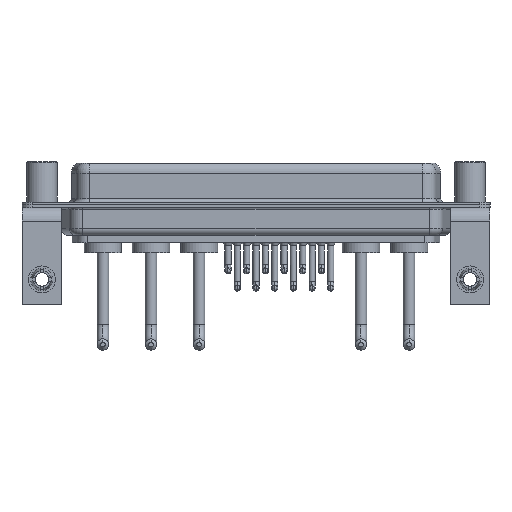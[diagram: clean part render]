
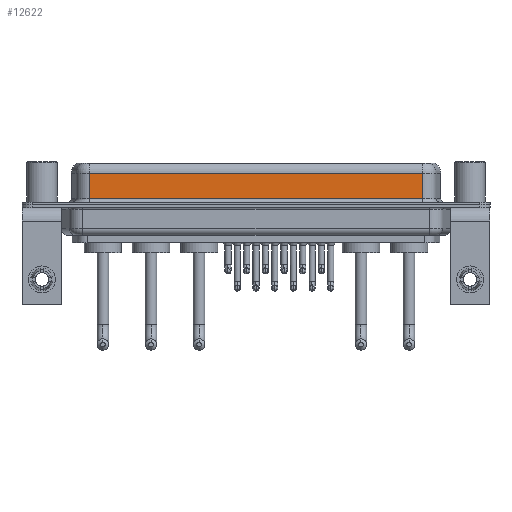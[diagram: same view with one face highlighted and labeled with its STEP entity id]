
A CAD part, front view. The second image highlights one B-rep face of the part: STEP entity #12622.
In plain terms, the highlighted planar face has unit normal (0, -1, 0).
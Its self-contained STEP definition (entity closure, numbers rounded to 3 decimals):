
#1350 = PLANE ( 'NONE',  #12972 ) ;
#1439 = ORIENTED_EDGE ( 'NONE', *, *, #18335, .T. ) ;
#1693 = CARTESIAN_POINT ( 'NONE',  ( 56.462, -3.95, 6.4 ) ) ;
#1895 = ORIENTED_EDGE ( 'NONE', *, *, #17856, .F. ) ;
#3363 = ORIENTED_EDGE ( 'NONE', *, *, #7314, .T. ) ;
#4393 = DIRECTION ( 'NONE',  ( -1., 0., 0. ) ) ;
#5036 = FACE_OUTER_BOUND ( 'NONE', #7839, .T. ) ;
#5553 = ORIENTED_EDGE ( 'NONE', *, *, #11568, .T. ) ;
#7024 = DIRECTION ( 'NONE',  ( 0., 0., 1. ) ) ;
#7314 = EDGE_CURVE ( 'NONE', #15462, #13961, #13745, .T. ) ;
#7839 = EDGE_LOOP ( 'NONE', ( #1895, #3363, #1439, #5553 ) ) ;
#8731 = VERTEX_POINT ( 'NONE', #11573 ) ;
#8867 = CARTESIAN_POINT ( 'NONE',  ( 56.462, -3.95, 6.4 ) ) ;
#10693 = CARTESIAN_POINT ( 'NONE',  ( 7.038, -3.95, 4.65 ) ) ;
#10932 = DIRECTION ( 'NONE',  ( 0., 1., 0. ) ) ;
#11375 = CARTESIAN_POINT ( 'NONE',  ( 7.038, -3.95, 0.9 ) ) ;
#11501 = CARTESIAN_POINT ( 'NONE',  ( 7.038, -3.95, 6.4 ) ) ;
#11568 = EDGE_CURVE ( 'NONE', #18239, #8731, #11777, .T. ) ;
#11573 = CARTESIAN_POINT ( 'NONE',  ( 56.462, -3.95, 0.9 ) ) ;
#11585 = CARTESIAN_POINT ( 'NONE',  ( 56.462, -3.95, 4.65 ) ) ;
#11657 = CARTESIAN_POINT ( 'NONE',  ( 56.462, -3.95, 0.9 ) ) ;
#11760 = VECTOR ( 'NONE', #17710, 1000. ) ;
#11777 = LINE ( 'NONE', #11657, #11760 ) ;
#11857 = DIRECTION ( 'NONE',  ( 0., 0., -1. ) ) ;
#12622 = ADVANCED_FACE ( 'NONE', ( #5036 ), #1350, .F. ) ;
#12972 = AXIS2_PLACEMENT_3D ( 'NONE', #8867, #10932, #7024 ) ;
#13231 = VECTOR ( 'NONE', #4393, 1000. ) ;
#13717 = LINE ( 'NONE', #11501, #23989 ) ;
#13745 = LINE ( 'NONE', #21306, #13231 ) ;
#13961 = VERTEX_POINT ( 'NONE', #10693 ) ;
#15462 = VERTEX_POINT ( 'NONE', #11585 ) ;
#17710 = DIRECTION ( 'NONE',  ( 1., 0., 0. ) ) ;
#17856 = EDGE_CURVE ( 'NONE', #15462, #8731, #18586, .T. ) ;
#18239 = VERTEX_POINT ( 'NONE', #11375 ) ;
#18335 = EDGE_CURVE ( 'NONE', #13961, #18239, #13717, .T. ) ;
#18586 = LINE ( 'NONE', #1693, #22801 ) ;
#21306 = CARTESIAN_POINT ( 'NONE',  ( 56.462, -3.95, 4.65 ) ) ;
#22533 = DIRECTION ( 'NONE',  ( 0., 0., -1. ) ) ;
#22801 = VECTOR ( 'NONE', #22533, 1000. ) ;
#23989 = VECTOR ( 'NONE', #11857, 1000. ) ;
